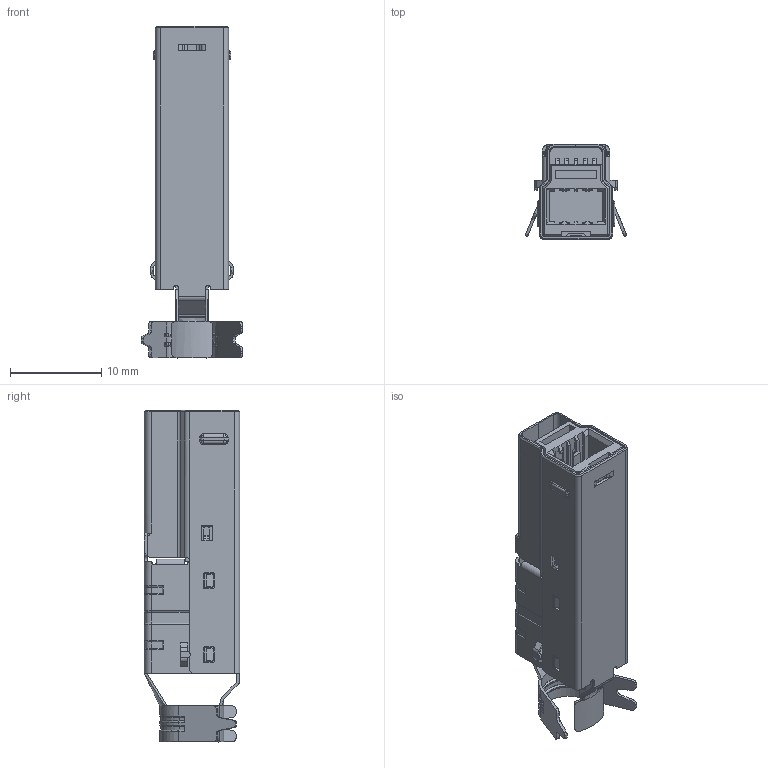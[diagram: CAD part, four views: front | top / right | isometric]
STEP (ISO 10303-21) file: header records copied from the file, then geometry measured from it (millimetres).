
FILE_DESCRIPTION (( 'STEP AP214' ), '1' );
FILE_NAME ('691F209-190-712.STEP', '2021-01-19T15:37:38', ( '' ), ( '' ), 'SwSTEP 2.0', 'SolidWorks 2020', '' );
FILE_SCHEMA (( 'AUTOMOTIVE_DESIGN' ));
Length unit declared in the file: millimetre
Products named in the file (5): 691F209-190-712; Contacts 691F209-X90-7XX; Shell 2 691F209-X90-7XX; Shell 1 691F209-X90-7XX; Insulator 691F209-X90-7XX_Blue
Assembly tree (4 placements, depth 2):
  691F209-190-712
    Insulator 691F209-X90-7XX_Blue
    Shell 2 691F209-X90-7XX
    Shell 1 691F209-X90-7XX
    Contacts 691F209-X90-7XX
Bounding box: 11.11 x 10.44 x 36.3 mm (x, y, z)
Volume: 808.9 mm3; surface area: 3749.7 mm2
Topology: 11 solids, 12 shells, 1480 faces, 4050 edges, 2544 vertices
Faces by surface type: plane 816, cylinder 525, bspline 118, cone 21
Entity records: 49330 total; most frequent: CARTESIAN_POINT 13028, ORIENTED_EDGE 8004, DIRECTION 6933, EDGE_CURVE 4002, VERTEX_POINT 2544, LINE 2541, VECTOR 2541, AXIS2_PLACEMENT_3D 2196
